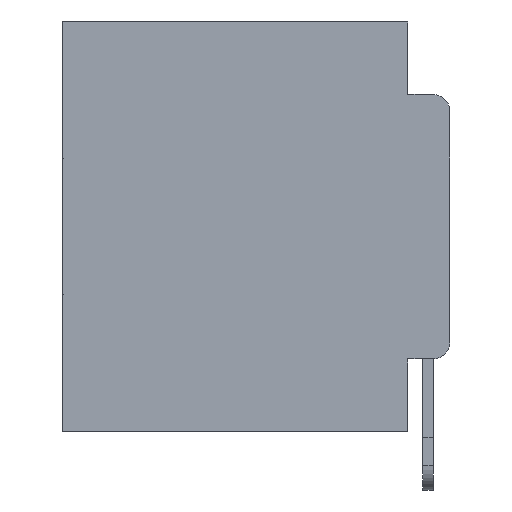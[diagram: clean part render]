
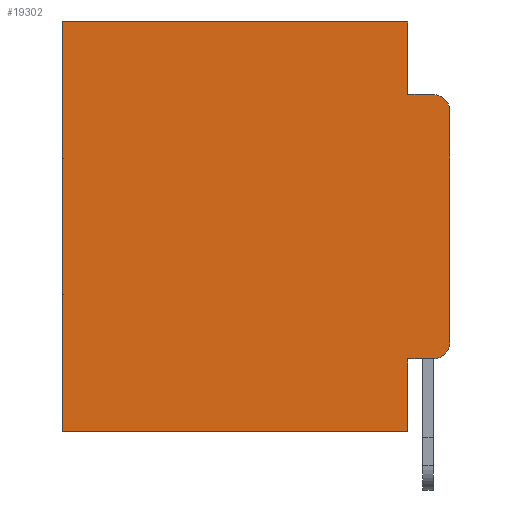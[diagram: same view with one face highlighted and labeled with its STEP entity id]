
A CAD part, left-side view. The second image highlights one B-rep face of the part: STEP entity #19302.
In plain terms, the highlighted planar face has unit normal (-1, 0, 0).
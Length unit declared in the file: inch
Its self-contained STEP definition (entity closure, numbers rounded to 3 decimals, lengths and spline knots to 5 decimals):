
#287 = VERTEX_POINT ( 'NONE', #12307 ) ;
#1898 = DIRECTION ( 'NONE',  ( 0., 0., -1. ) ) ;
#2072 = VERTEX_POINT ( 'NONE', #16453 ) ;
#2125 = DIRECTION ( 'NONE',  ( 0., 0., -1. ) ) ;
#2254 = EDGE_CURVE ( 'NONE', #2072, #17003, #15212, .T. ) ;
#2560 = DIRECTION ( 'NONE',  ( 0., 0., -1. ) ) ;
#2955 = VERTEX_POINT ( 'NONE', #10730 ) ;
#3404 = DIRECTION ( 'NONE',  ( 1., 0., 0. ) ) ;
#3698 = EDGE_CURVE ( 'NONE', #6410, #2955, #24296, .T. ) ;
#3940 = EDGE_CURVE ( 'NONE', #17003, #10151, #17639, .T. ) ;
#4849 = VECTOR ( 'NONE', #8199, 39.37008 ) ;
#5314 = ORIENTED_EDGE ( 'NONE', *, *, #3940, .F. ) ;
#5315 = LINE ( 'NONE', #7772, #17343 ) ;
#5690 = EDGE_CURVE ( 'NONE', #2072, #10393, #16057, .T. ) ;
#5731 = ORIENTED_EDGE ( 'NONE', *, *, #8453, .F. ) ;
#6410 = VERTEX_POINT ( 'NONE', #8051 ) ;
#6480 = AXIS2_PLACEMENT_3D ( 'NONE', #17902, #3404, #20189 ) ;
#7099 = DIRECTION ( 'NONE',  ( 0., 1., 0. ) ) ;
#7108 = LINE ( 'NONE', #27234, #12126 ) ;
#7240 = CARTESIAN_POINT ( 'NONE',  ( 0.298, 0.051, 0. ) ) ;
#7772 = CARTESIAN_POINT ( 'NONE',  ( 0.298, 0., 0. ) ) ;
#8024 = VECTOR ( 'NONE', #9059, 39.37008 ) ;
#8051 = CARTESIAN_POINT ( 'NONE',  ( 0.298, 0.02, -0.4115 ) ) ;
#8199 = DIRECTION ( 'NONE',  ( 0., -1., 0. ) ) ;
#8453 = EDGE_CURVE ( 'NONE', #26284, #287, #29617, .T. ) ;
#8604 = EDGE_CURVE ( 'NONE', #9116, #2955, #5315, .T. ) ;
#8857 = EDGE_CURVE ( 'NONE', #9116, #10151, #9267, .T. ) ;
#9059 = DIRECTION ( 'NONE',  ( 0., -1., 0. ) ) ;
#9116 = VERTEX_POINT ( 'NONE', #26678 ) ;
#9267 = CIRCLE ( 'NONE', #15155, 0.02 ) ;
#9292 = ORIENTED_EDGE ( 'NONE', *, *, #5690, .T. ) ;
#9482 = VECTOR ( 'NONE', #2125, 39.37008 ) ;
#9655 = EDGE_CURVE ( 'NONE', #14773, #6410, #15106, .T. ) ;
#10151 = VERTEX_POINT ( 'NONE', #22970 ) ;
#10393 = VERTEX_POINT ( 'NONE', #15190 ) ;
#10730 = CARTESIAN_POINT ( 'NONE',  ( 0.298, 0., -0.3915 ) ) ;
#11395 = DIRECTION ( 'NONE',  ( 0., 0., -1. ) ) ;
#11527 = DIRECTION ( 'NONE',  ( -1., 0., 0. ) ) ;
#12126 = VECTOR ( 'NONE', #11395, 39.37008 ) ;
#12307 = CARTESIAN_POINT ( 'NONE',  ( 0.298, 0.473, -0.5 ) ) ;
#12910 = CARTESIAN_POINT ( 'NONE',  ( 0.298, 0.051, -0.4115 ) ) ;
#12967 = CARTESIAN_POINT ( 'NONE',  ( 0.298, 0.051, -0.0885 ) ) ;
#13059 = ORIENTED_EDGE ( 'NONE', *, *, #20857, .F. ) ;
#14122 = EDGE_LOOP ( 'NONE', ( #14497, #15892, #5314, #30647, #9292, #22301, #5731, #13059, #15204, #23388 ) ) ;
#14497 = ORIENTED_EDGE ( 'NONE', *, *, #8604, .F. ) ;
#14773 = VERTEX_POINT ( 'NONE', #12910 ) ;
#15021 = LINE ( 'NONE', #16806, #9482 ) ;
#15106 = LINE ( 'NONE', #22909, #8024 ) ;
#15155 = AXIS2_PLACEMENT_3D ( 'NONE', #25118, #11527, #27362 ) ;
#15190 = CARTESIAN_POINT ( 'NONE',  ( 0.298, 0.473, 0. ) ) ;
#15204 = ORIENTED_EDGE ( 'NONE', *, *, #9655, .T. ) ;
#15212 = LINE ( 'NONE', #7240, #26468 ) ;
#15397 = CARTESIAN_POINT ( 'NONE',  ( 0.298, 0.051, -0.5 ) ) ;
#15892 = ORIENTED_EDGE ( 'NONE', *, *, #8857, .T. ) ;
#16057 = LINE ( 'NONE', #27788, #27321 ) ;
#16453 = CARTESIAN_POINT ( 'NONE',  ( 0.298, 0.051, 0. ) ) ;
#16471 = FACE_OUTER_BOUND ( 'NONE', #14122, .T. ) ;
#16598 = DIRECTION ( 'NONE',  ( -1., 0., 0. ) ) ;
#16702 = DIRECTION ( 'NONE',  ( 0., 0., -1. ) ) ;
#16806 = CARTESIAN_POINT ( 'NONE',  ( 0.298, 0.473, 0. ) ) ;
#17003 = VERTEX_POINT ( 'NONE', #19908 ) ;
#17343 = VECTOR ( 'NONE', #2560, 39.37008 ) ;
#17639 = LINE ( 'NONE', #12967, #4849 ) ;
#17902 = CARTESIAN_POINT ( 'NONE',  ( 0.298, 0., 0. ) ) ;
#19302 = ADVANCED_FACE ( 'NONE', ( #16471 ), #24570, .F. ) ;
#19908 = CARTESIAN_POINT ( 'NONE',  ( 0.298, 0.051, -0.0885 ) ) ;
#20189 = DIRECTION ( 'NONE',  ( 0., 0., -1. ) ) ;
#20857 = EDGE_CURVE ( 'NONE', #14773, #26284, #7108, .T. ) ;
#21156 = DIRECTION ( 'NONE',  ( 0., 1., 0. ) ) ;
#22301 = ORIENTED_EDGE ( 'NONE', *, *, #23675, .T. ) ;
#22455 = AXIS2_PLACEMENT_3D ( 'NONE', #30025, #16598, #1898 ) ;
#22909 = CARTESIAN_POINT ( 'NONE',  ( 0.298, 0.051, -0.4115 ) ) ;
#22970 = CARTESIAN_POINT ( 'NONE',  ( 0.298, 0.02, -0.0885 ) ) ;
#23388 = ORIENTED_EDGE ( 'NONE', *, *, #3698, .T. ) ;
#23675 = EDGE_CURVE ( 'NONE', #10393, #287, #15021, .T. ) ;
#24296 = CIRCLE ( 'NONE', #22455, 0.02 ) ;
#24570 = PLANE ( 'NONE',  #6480 ) ;
#25118 = CARTESIAN_POINT ( 'NONE',  ( 0.298, 0.02, -0.1085 ) ) ;
#26284 = VERTEX_POINT ( 'NONE', #15397 ) ;
#26468 = VECTOR ( 'NONE', #16702, 39.37008 ) ;
#26678 = CARTESIAN_POINT ( 'NONE',  ( 0.298, 0., -0.1085 ) ) ;
#27234 = CARTESIAN_POINT ( 'NONE',  ( 0.298, 0.051, 0. ) ) ;
#27321 = VECTOR ( 'NONE', #7099, 39.37008 ) ;
#27362 = DIRECTION ( 'NONE',  ( 0., 0., -1. ) ) ;
#27788 = CARTESIAN_POINT ( 'NONE',  ( 0.298, 0., 0. ) ) ;
#29617 = LINE ( 'NONE', #30016, #30325 ) ;
#30016 = CARTESIAN_POINT ( 'NONE',  ( 0.298, 0., -0.5 ) ) ;
#30025 = CARTESIAN_POINT ( 'NONE',  ( 0.298, 0.02, -0.3915 ) ) ;
#30325 = VECTOR ( 'NONE', #21156, 39.37008 ) ;
#30647 = ORIENTED_EDGE ( 'NONE', *, *, #2254, .F. ) ;
